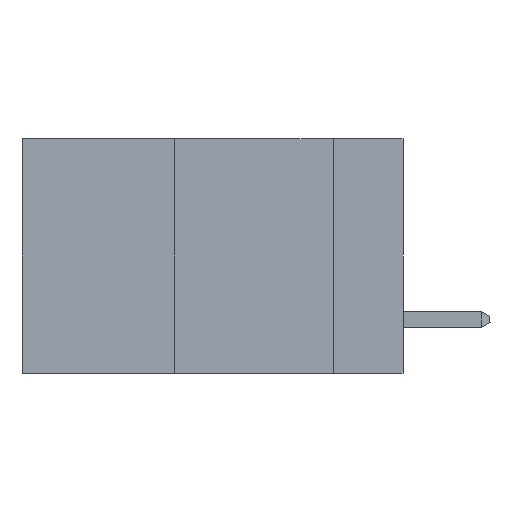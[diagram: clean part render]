
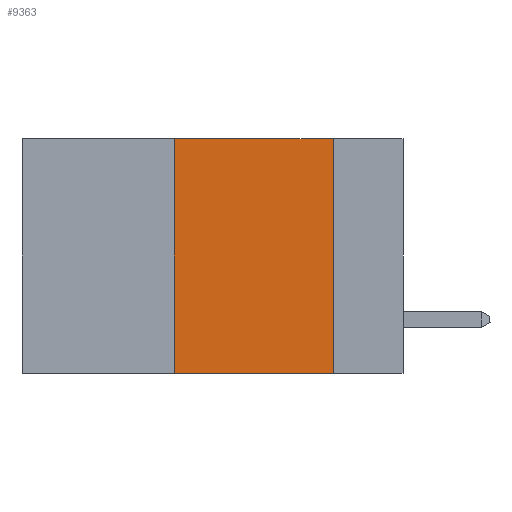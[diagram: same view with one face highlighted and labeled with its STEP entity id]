
A CAD part, left-side view. The second image highlights one B-rep face of the part: STEP entity #9363.
In plain terms, the highlighted planar face has unit normal (-1, 0, 0).
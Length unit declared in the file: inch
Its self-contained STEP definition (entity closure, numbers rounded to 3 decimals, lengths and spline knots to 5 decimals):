
#61 = VERTEX_POINT ( 'NONE', #4981 ) ;
#294 = CARTESIAN_POINT ( 'NONE',  ( 0., 0.6, 0. ) ) ;
#643 = ORIENTED_EDGE ( 'NONE', *, *, #9492, .F. ) ;
#964 = EDGE_LOOP ( 'NONE', ( #14954, #11406, #643, #12926 ) ) ;
#1100 = LINE ( 'NONE', #3836, #10477 ) ;
#1616 = DIRECTION ( 'NONE',  ( 0., 0., -1. ) ) ;
#2555 = CARTESIAN_POINT ( 'NONE',  ( 0., 0.11, -0.37 ) ) ;
#3815 = CARTESIAN_POINT ( 'NONE',  ( 0., 0.6, 0. ) ) ;
#3836 = CARTESIAN_POINT ( 'NONE',  ( 0., 0.6, -0.37 ) ) ;
#3890 = DIRECTION ( 'NONE',  ( 0., -1., 0. ) ) ;
#3986 = LINE ( 'NONE', #3815, #13580 ) ;
#4606 = DIRECTION ( 'NONE',  ( 0., 0., -1. ) ) ;
#4762 = VERTEX_POINT ( 'NONE', #6045 ) ;
#4981 = CARTESIAN_POINT ( 'NONE',  ( 0., 0.36, 0. ) ) ;
#5717 = FACE_OUTER_BOUND ( 'NONE', #964, .T. ) ;
#5818 = LINE ( 'NONE', #15299, #12124 ) ;
#6045 = CARTESIAN_POINT ( 'NONE',  ( 0., 0.11, 0. ) ) ;
#6501 = AXIS2_PLACEMENT_3D ( 'NONE', #294, #9005, #1616 ) ;
#7075 = DIRECTION ( 'NONE',  ( 0., 0., 1. ) ) ;
#7813 = PLANE ( 'NONE',  #6501 ) ;
#7927 = EDGE_CURVE ( 'NONE', #61, #4762, #3986, .T. ) ;
#9005 = DIRECTION ( 'NONE',  ( 1., 0., 0. ) ) ;
#9363 = ADVANCED_FACE ( 'NONE', ( #5717 ), #7813, .F. ) ;
#9492 = EDGE_CURVE ( 'NONE', #9625, #61, #15693, .T. ) ;
#9625 = VERTEX_POINT ( 'NONE', #15477 ) ;
#10477 = VECTOR ( 'NONE', #3890, 39.37008 ) ;
#11056 = DIRECTION ( 'NONE',  ( 0., -1., 0. ) ) ;
#11406 = ORIENTED_EDGE ( 'NONE', *, *, #7927, .F. ) ;
#12124 = VECTOR ( 'NONE', #4606, 39.37008 ) ;
#12216 = VECTOR ( 'NONE', #7075, 39.37008 ) ;
#12901 = CARTESIAN_POINT ( 'NONE',  ( 0., 0.36, 0. ) ) ;
#12926 = ORIENTED_EDGE ( 'NONE', *, *, #14193, .T. ) ;
#13580 = VECTOR ( 'NONE', #11056, 39.37008 ) ;
#13895 = EDGE_CURVE ( 'NONE', #4762, #15348, #5818, .T. ) ;
#14193 = EDGE_CURVE ( 'NONE', #9625, #15348, #1100, .T. ) ;
#14954 = ORIENTED_EDGE ( 'NONE', *, *, #13895, .F. ) ;
#15299 = CARTESIAN_POINT ( 'NONE',  ( 0., 0.11, 0. ) ) ;
#15348 = VERTEX_POINT ( 'NONE', #2555 ) ;
#15477 = CARTESIAN_POINT ( 'NONE',  ( 0., 0.36, -0.37 ) ) ;
#15693 = LINE ( 'NONE', #12901, #12216 ) ;
